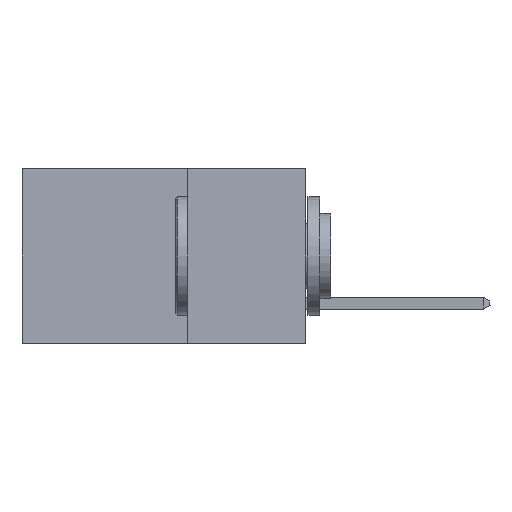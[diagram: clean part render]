
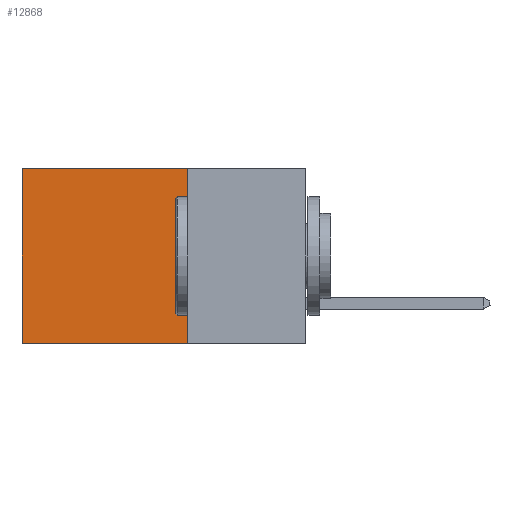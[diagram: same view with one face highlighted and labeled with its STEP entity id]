
A CAD part, left-side view. The second image highlights one B-rep face of the part: STEP entity #12868.
In plain terms, the highlighted planar face has unit normal (-1, 0, 0).
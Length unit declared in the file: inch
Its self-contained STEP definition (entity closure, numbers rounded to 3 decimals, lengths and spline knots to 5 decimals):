
#1243 = AXIS2_PLACEMENT_3D ( 'NONE', #6492, #4494, #2918 ) ;
#1648 = CARTESIAN_POINT ( 'NONE',  ( 0.298, 0.6, -0.37 ) ) ;
#1711 = FACE_OUTER_BOUND ( 'NONE', #7183, .T. ) ;
#1825 = CARTESIAN_POINT ( 'NONE',  ( 0.298, 0.6, 0. ) ) ;
#2700 = EDGE_CURVE ( 'NONE', #7947, #18668, #16032, .T. ) ;
#2918 = DIRECTION ( 'NONE',  ( 0., 0., -1. ) ) ;
#3250 = ORIENTED_EDGE ( 'NONE', *, *, #5977, .F. ) ;
#4331 = EDGE_CURVE ( 'NONE', #14258, #18668, #13451, .T. ) ;
#4494 = DIRECTION ( 'NONE',  ( 1., 0., 0. ) ) ;
#5698 = DIRECTION ( 'NONE',  ( 0., 0., -1. ) ) ;
#5977 = EDGE_CURVE ( 'NONE', #19548, #7947, #9867, .T. ) ;
#6492 = CARTESIAN_POINT ( 'NONE',  ( 0.298, 0.25, 0. ) ) ;
#6620 = CARTESIAN_POINT ( 'NONE',  ( 0.298, 0.25, -0.37 ) ) ;
#6741 = CARTESIAN_POINT ( 'NONE',  ( 0.298, 0.25, -0.37 ) ) ;
#7183 = EDGE_LOOP ( 'NONE', ( #10526, #22533, #3250, #12804 ) ) ;
#7947 = VERTEX_POINT ( 'NONE', #6620 ) ;
#9503 = VECTOR ( 'NONE', #14500, 39.37008 ) ;
#9867 = LINE ( 'NONE', #20184, #10685 ) ;
#10126 = DIRECTION ( 'NONE',  ( 0., 1., 0. ) ) ;
#10526 = ORIENTED_EDGE ( 'NONE', *, *, #4331, .T. ) ;
#10685 = VECTOR ( 'NONE', #5698, 39.37008 ) ;
#11640 = CARTESIAN_POINT ( 'NONE',  ( 0.298, 0.25, 0. ) ) ;
#12804 = ORIENTED_EDGE ( 'NONE', *, *, #14087, .T. ) ;
#12868 = ADVANCED_FACE ( 'NONE', ( #1711 ), #17212, .F. ) ;
#13451 = LINE ( 'NONE', #1825, #9503 ) ;
#14040 = VECTOR ( 'NONE', #10126, 39.37008 ) ;
#14087 = EDGE_CURVE ( 'NONE', #19548, #14258, #18546, .T. ) ;
#14258 = VERTEX_POINT ( 'NONE', #21336 ) ;
#14500 = DIRECTION ( 'NONE',  ( 0., 0., -1. ) ) ;
#15881 = DIRECTION ( 'NONE',  ( 0., 1., 0. ) ) ;
#16032 = LINE ( 'NONE', #6741, #17167 ) ;
#17167 = VECTOR ( 'NONE', #15881, 39.37008 ) ;
#17212 = PLANE ( 'NONE',  #1243 ) ;
#18546 = LINE ( 'NONE', #20747, #14040 ) ;
#18668 = VERTEX_POINT ( 'NONE', #1648 ) ;
#19548 = VERTEX_POINT ( 'NONE', #11640 ) ;
#20184 = CARTESIAN_POINT ( 'NONE',  ( 0.298, 0.25, 0. ) ) ;
#20747 = CARTESIAN_POINT ( 'NONE',  ( 0.298, 0.25, 0. ) ) ;
#21336 = CARTESIAN_POINT ( 'NONE',  ( 0.298, 0.6, 0. ) ) ;
#22533 = ORIENTED_EDGE ( 'NONE', *, *, #2700, .F. ) ;
